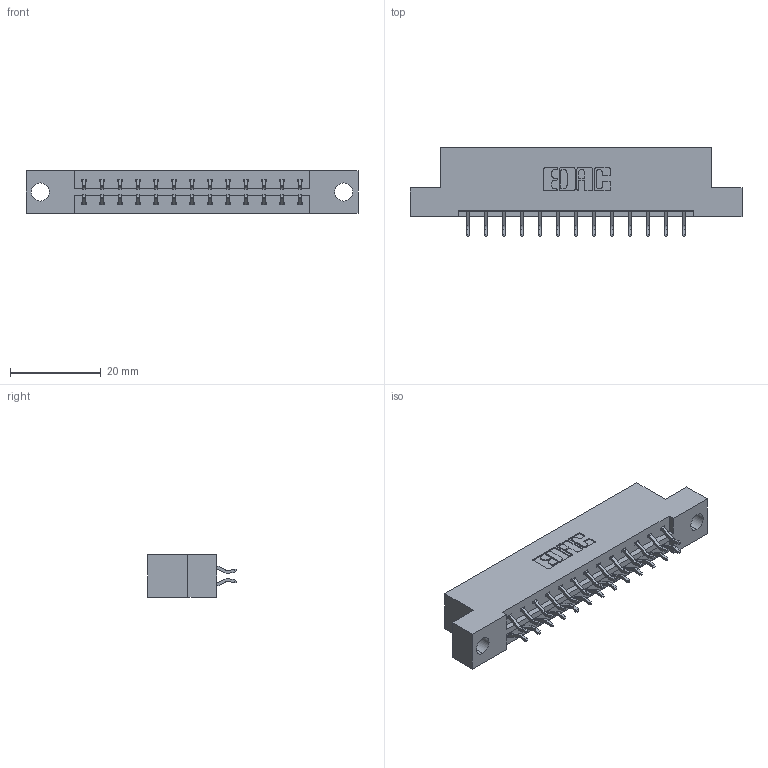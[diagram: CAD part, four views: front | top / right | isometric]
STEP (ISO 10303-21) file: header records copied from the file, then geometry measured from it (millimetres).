
FILE_DESCRIPTION (( 'STEP AP203' ), '1' );
FILE_NAME ('333-026-556-204.STEP', '2018-08-02T13:20:50', ( '' ), ( '' ), 'SwSTEP 2.0', 'SolidWorks 2016', '' );
FILE_SCHEMA (( 'CONFIG_CONTROL_DESIGN' ));
Length unit declared in the file: inch
Products named in the file (3): 333 Part_Flush - .156 Dia - TH; 345-292-001_556 Tail; 333-026-556-204
Assembly tree (27 placements, depth 2):
  333-026-556-204
    333 Part_Flush - .156 Dia - TH
    345-292-001_556 Tail  x26
Bounding box: 73.05 x 19.57 x 9.4 mm (x, y, z)
Volume: 7097.9 mm3; surface area: 7853.7 mm2
Topology: 27 solids, 27 shells, 1622 faces, 4809 edges, 3170 vertices
Faces by surface type: plane 1110, cylinder 512
Entity records: 12337 total; most frequent: CARTESIAN_POINT 2094, ORIENTED_EDGE 2018, DIRECTION 1829, EDGE_CURVE 1009, VECTOR 873, LINE 873, VERTEX_POINT 670, AXIS2_PLACEMENT_3D 478
